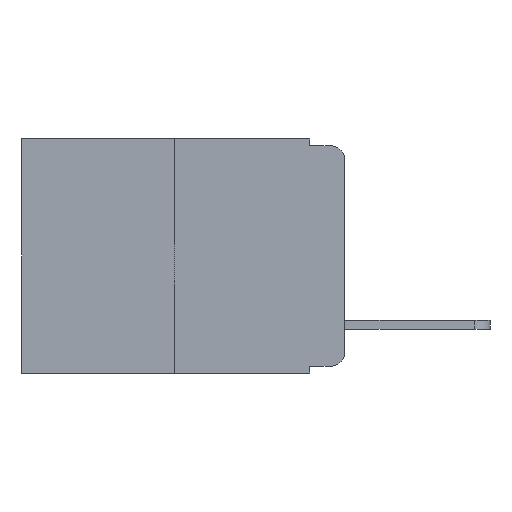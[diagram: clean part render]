
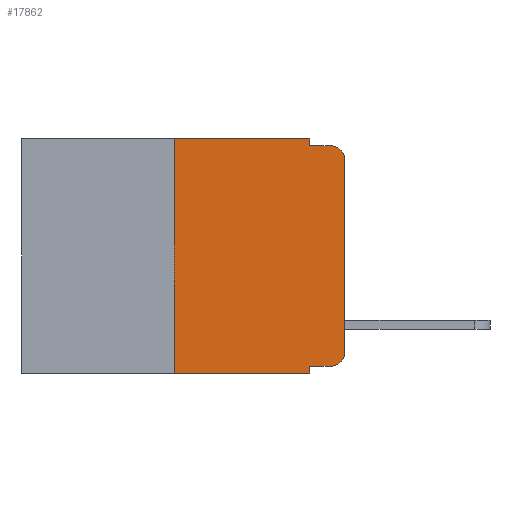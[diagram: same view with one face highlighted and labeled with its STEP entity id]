
A CAD part, left-side view. The second image highlights one B-rep face of the part: STEP entity #17862.
In plain terms, the highlighted planar face has unit normal (-1, 0, 0).
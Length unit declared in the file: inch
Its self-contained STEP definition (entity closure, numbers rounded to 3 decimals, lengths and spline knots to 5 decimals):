
#2 = PLANE ( 'NONE',  #4835 ) ;
#314 = CARTESIAN_POINT ( 'NONE',  ( 0., 0.051, 0. ) ) ;
#335 = LINE ( 'NONE', #8483, #4203 ) ;
#395 = CARTESIAN_POINT ( 'NONE',  ( 0., 0.051, 0. ) ) ;
#814 = DIRECTION ( 'NONE',  ( -1., 0., 0. ) ) ;
#1481 = LINE ( 'NONE', #395, #14517 ) ;
#1724 = CARTESIAN_POINT ( 'NONE',  ( 0., 0.051, -0.343 ) ) ;
#1806 = DIRECTION ( 'NONE',  ( 1., 0., 0. ) ) ;
#2005 = CARTESIAN_POINT ( 'NONE',  ( 0., 0.051, -0.01 ) ) ;
#2010 = AXIS2_PLACEMENT_3D ( 'NONE', #10557, #814, #12059 ) ;
#2016 = LINE ( 'NONE', #16019, #10160 ) ;
#2125 = VERTEX_POINT ( 'NONE', #15286 ) ;
#2472 = CARTESIAN_POINT ( 'NONE',  ( 0., 0.051, -0.333 ) ) ;
#3027 = VERTEX_POINT ( 'NONE', #11356 ) ;
#3194 = CARTESIAN_POINT ( 'NONE',  ( 0., 0.473, 0. ) ) ;
#3766 = DIRECTION ( 'NONE',  ( -1., 0., 0. ) ) ;
#3773 = CARTESIAN_POINT ( 'NONE',  ( 0., 0.02, -0.333 ) ) ;
#4203 = VECTOR ( 'NONE', #17121, 39.37008 ) ;
#4835 = AXIS2_PLACEMENT_3D ( 'NONE', #18295, #1806, #12918 ) ;
#5820 = CARTESIAN_POINT ( 'NONE',  ( 0., 0.25, 0. ) ) ;
#6237 = ORIENTED_EDGE ( 'NONE', *, *, #12814, .T. ) ;
#6287 = VERTEX_POINT ( 'NONE', #1724 ) ;
#6295 = ORIENTED_EDGE ( 'NONE', *, *, #12844, .T. ) ;
#6451 = ORIENTED_EDGE ( 'NONE', *, *, #12850, .F. ) ;
#6581 = VECTOR ( 'NONE', #13151, 39.37008 ) ;
#6588 = DIRECTION ( 'NONE',  ( 0., -1., 0. ) ) ;
#7095 = VECTOR ( 'NONE', #17234, 39.37008 ) ;
#7215 = DIRECTION ( 'NONE',  ( 0., 0., -1. ) ) ;
#7284 = ORIENTED_EDGE ( 'NONE', *, *, #12873, .F. ) ;
#7410 = ORIENTED_EDGE ( 'NONE', *, *, #11824, .F. ) ;
#7644 = ORIENTED_EDGE ( 'NONE', *, *, #12879, .F. ) ;
#7963 = ORIENTED_EDGE ( 'NONE', *, *, #12349, .T. ) ;
#8440 = ORIENTED_EDGE ( 'NONE', *, *, #12898, .F. ) ;
#8483 = CARTESIAN_POINT ( 'NONE',  ( 0., 0., 0. ) ) ;
#8525 = LINE ( 'NONE', #2005, #7095 ) ;
#8734 = DIRECTION ( 'NONE',  ( 0., 0., 1. ) ) ;
#9486 = ORIENTED_EDGE ( 'NONE', *, *, #12901, .T. ) ;
#9606 = ORIENTED_EDGE ( 'NONE', *, *, #12905, .T. ) ;
#9664 = VECTOR ( 'NONE', #11731, 39.37008 ) ;
#10160 = VECTOR ( 'NONE', #8734, 39.37008 ) ;
#10318 = CARTESIAN_POINT ( 'NONE',  ( 0., 0.25, -0.343 ) ) ;
#10557 = CARTESIAN_POINT ( 'NONE',  ( 0., 0.02, -0.313 ) ) ;
#11091 = LINE ( 'NONE', #314, #6581 ) ;
#11341 = LINE ( 'NONE', #3194, #14753 ) ;
#11356 = CARTESIAN_POINT ( 'NONE',  ( 0., 0.051, 0. ) ) ;
#11542 = CIRCLE ( 'NONE', #19305, 0.02 ) ;
#11731 = DIRECTION ( 'NONE',  ( 0., -1., 0. ) ) ;
#11800 = CARTESIAN_POINT ( 'NONE',  ( 0., 0.051, -0.01 ) ) ;
#11824 = EDGE_CURVE ( 'NONE', #13546, #3027, #11341, .T. ) ;
#12059 = DIRECTION ( 'NONE',  ( 0., 0., -1. ) ) ;
#12349 = EDGE_CURVE ( 'NONE', #18442, #6287, #12468, .T. ) ;
#12468 = LINE ( 'NONE', #18121, #15383 ) ;
#12732 = VERTEX_POINT ( 'NONE', #15535 ) ;
#12814 = EDGE_CURVE ( 'NONE', #12732, #16197, #335, .T. ) ;
#12844 = EDGE_CURVE ( 'NONE', #16197, #19175, #11542, .T. ) ;
#12850 = EDGE_CURVE ( 'NONE', #16636, #19175, #8525, .T. ) ;
#12873 = EDGE_CURVE ( 'NONE', #3027, #16636, #11091, .T. ) ;
#12879 = EDGE_CURVE ( 'NONE', #18442, #13546, #2016, .T. ) ;
#12898 = EDGE_CURVE ( 'NONE', #2125, #6287, #1481, .T. ) ;
#12901 = EDGE_CURVE ( 'NONE', #2125, #14736, #14077, .T. ) ;
#12905 = EDGE_CURVE ( 'NONE', #14736, #12732, #17689, .T. ) ;
#12918 = DIRECTION ( 'NONE',  ( 0., 0., -1. ) ) ;
#13090 = CARTESIAN_POINT ( 'NONE',  ( 0., 0.02, -0.03 ) ) ;
#13151 = DIRECTION ( 'NONE',  ( 0., 0., -1. ) ) ;
#13546 = VERTEX_POINT ( 'NONE', #5820 ) ;
#14077 = LINE ( 'NONE', #2472, #9664 ) ;
#14301 = EDGE_LOOP ( 'NONE', ( #6237, #6295, #6451, #7284, #7410, #7644, #7963, #8440, #9486, #9606 ) ) ;
#14517 = VECTOR ( 'NONE', #7215, 39.37008 ) ;
#14538 = DIRECTION ( 'NONE',  ( 0., 0., -1. ) ) ;
#14736 = VERTEX_POINT ( 'NONE', #3773 ) ;
#14753 = VECTOR ( 'NONE', #18140, 39.37008 ) ;
#15286 = CARTESIAN_POINT ( 'NONE',  ( 0., 0.051, -0.333 ) ) ;
#15383 = VECTOR ( 'NONE', #6588, 39.37008 ) ;
#15535 = CARTESIAN_POINT ( 'NONE',  ( 0., 0., -0.313 ) ) ;
#16019 = CARTESIAN_POINT ( 'NONE',  ( 0., 0.25, 0. ) ) ;
#16197 = VERTEX_POINT ( 'NONE', #19290 ) ;
#16498 = CARTESIAN_POINT ( 'NONE',  ( 0., 0.02, -0.01 ) ) ;
#16636 = VERTEX_POINT ( 'NONE', #11800 ) ;
#17121 = DIRECTION ( 'NONE',  ( 0., 0., 1. ) ) ;
#17234 = DIRECTION ( 'NONE',  ( 0., -1., 0. ) ) ;
#17689 = CIRCLE ( 'NONE', #2010, 0.02 ) ;
#17862 = ADVANCED_FACE ( 'NONE', ( #18153 ), #2, .F. ) ;
#18121 = CARTESIAN_POINT ( 'NONE',  ( 0., 0.473, -0.343 ) ) ;
#18140 = DIRECTION ( 'NONE',  ( 0., -1., 0. ) ) ;
#18153 = FACE_OUTER_BOUND ( 'NONE', #14301, .T. ) ;
#18295 = CARTESIAN_POINT ( 'NONE',  ( 0., 0.473, 0. ) ) ;
#18442 = VERTEX_POINT ( 'NONE', #10318 ) ;
#19175 = VERTEX_POINT ( 'NONE', #16498 ) ;
#19290 = CARTESIAN_POINT ( 'NONE',  ( 0., 0., -0.03 ) ) ;
#19305 = AXIS2_PLACEMENT_3D ( 'NONE', #13090, #3766, #14538 ) ;
